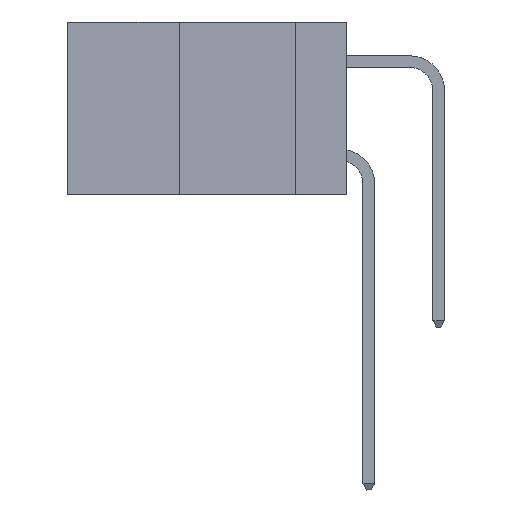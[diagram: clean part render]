
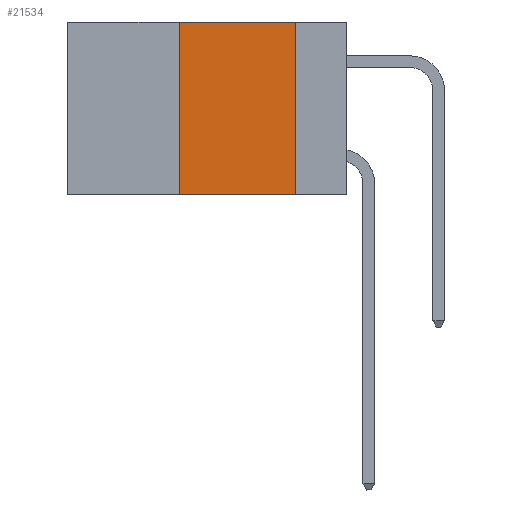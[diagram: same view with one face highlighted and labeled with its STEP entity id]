
A CAD part, left-side view. The second image highlights one B-rep face of the part: STEP entity #21534.
In plain terms, the highlighted planar face has unit normal (-1, 0, 0).
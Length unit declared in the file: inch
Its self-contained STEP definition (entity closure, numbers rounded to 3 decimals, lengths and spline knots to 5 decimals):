
#375 = ORIENTED_EDGE ( 'NONE', *, *, #13717, .F. ) ;
#658 = DIRECTION ( 'NONE',  ( 1., 0., 0. ) ) ;
#1087 = VECTOR ( 'NONE', #9790, 39.37008 ) ;
#1361 = DIRECTION ( 'NONE',  ( 0., -1., 0. ) ) ;
#1529 = FACE_OUTER_BOUND ( 'NONE', #16379, .T. ) ;
#1543 = VERTEX_POINT ( 'NONE', #18006 ) ;
#1761 = CARTESIAN_POINT ( 'NONE',  ( 0., 0.36, 0. ) ) ;
#4073 = EDGE_CURVE ( 'NONE', #14890, #23038, #21929, .T. ) ;
#5937 = LINE ( 'NONE', #21464, #22378 ) ;
#5939 = ORIENTED_EDGE ( 'NONE', *, *, #4073, .F. ) ;
#7453 = EDGE_CURVE ( 'NONE', #1543, #15245, #23444, .T. ) ;
#8240 = DIRECTION ( 'NONE',  ( 0., 0., 1. ) ) ;
#9314 = CARTESIAN_POINT ( 'NONE',  ( 0., 0.11, 0. ) ) ;
#9638 = DIRECTION ( 'NONE',  ( 0., 0., -1. ) ) ;
#9790 = DIRECTION ( 'NONE',  ( 0., -1., 0. ) ) ;
#9824 = ORIENTED_EDGE ( 'NONE', *, *, #17868, .T. ) ;
#10211 = CARTESIAN_POINT ( 'NONE',  ( 0., 0.11, -0.37 ) ) ;
#13123 = CARTESIAN_POINT ( 'NONE',  ( 0., 0.36, -0.37 ) ) ;
#13390 = DIRECTION ( 'NONE',  ( 0., 0., -1. ) ) ;
#13698 = LINE ( 'NONE', #20841, #1087 ) ;
#13717 = EDGE_CURVE ( 'NONE', #23038, #1543, #13698, .T. ) ;
#14890 = VERTEX_POINT ( 'NONE', #13123 ) ;
#15245 = VERTEX_POINT ( 'NONE', #10211 ) ;
#15943 = AXIS2_PLACEMENT_3D ( 'NONE', #19149, #658, #13390 ) ;
#16379 = EDGE_LOOP ( 'NONE', ( #20133, #375, #5939, #9824 ) ) ;
#16585 = VECTOR ( 'NONE', #9638, 39.37008 ) ;
#17868 = EDGE_CURVE ( 'NONE', #14890, #15245, #5937, .T. ) ;
#18006 = CARTESIAN_POINT ( 'NONE',  ( 0., 0.11, 0. ) ) ;
#19149 = CARTESIAN_POINT ( 'NONE',  ( 0., 0.6, 0. ) ) ;
#19697 = CARTESIAN_POINT ( 'NONE',  ( 0., 0.36, 0. ) ) ;
#19920 = VECTOR ( 'NONE', #8240, 39.37008 ) ;
#20133 = ORIENTED_EDGE ( 'NONE', *, *, #7453, .F. ) ;
#20841 = CARTESIAN_POINT ( 'NONE',  ( 0., 0.6, 0. ) ) ;
#21464 = CARTESIAN_POINT ( 'NONE',  ( 0., 0.6, -0.37 ) ) ;
#21534 = ADVANCED_FACE ( 'NONE', ( #1529 ), #22516, .F. ) ;
#21929 = LINE ( 'NONE', #19697, #19920 ) ;
#22378 = VECTOR ( 'NONE', #1361, 39.37008 ) ;
#22516 = PLANE ( 'NONE',  #15943 ) ;
#23038 = VERTEX_POINT ( 'NONE', #1761 ) ;
#23444 = LINE ( 'NONE', #9314, #16585 ) ;
